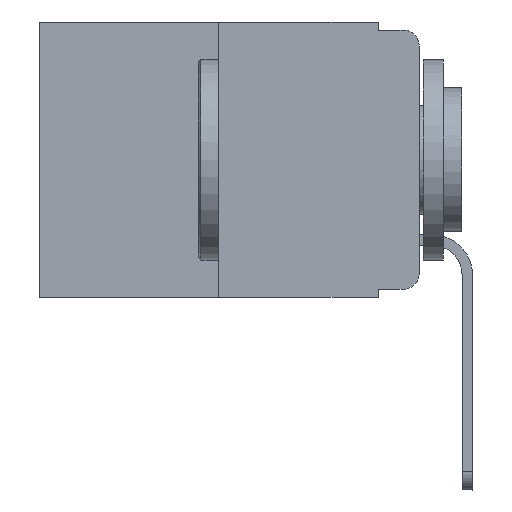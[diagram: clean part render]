
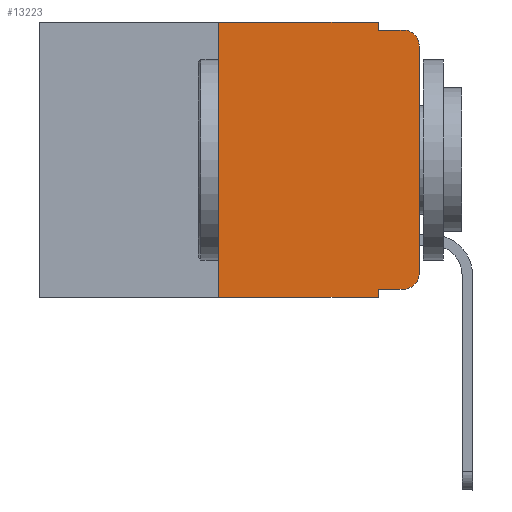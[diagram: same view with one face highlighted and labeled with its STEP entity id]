
A CAD part, left-side view. The second image highlights one B-rep face of the part: STEP entity #13223.
In plain terms, the highlighted planar face has unit normal (-1, 0, 0).
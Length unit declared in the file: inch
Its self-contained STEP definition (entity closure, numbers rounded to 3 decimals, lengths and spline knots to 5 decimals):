
#84 = CARTESIAN_POINT ( 'NONE',  ( 0., 0.02, -0.313 ) ) ;
#465 = ORIENTED_EDGE ( 'NONE', *, *, #11410, .T. ) ;
#489 = AXIS2_PLACEMENT_3D ( 'NONE', #3176, #11035, #1625 ) ;
#527 = EDGE_CURVE ( 'NONE', #16009, #16680, #5585, .T. ) ;
#617 = VERTEX_POINT ( 'NONE', #17067 ) ;
#781 = EDGE_CURVE ( 'NONE', #16009, #13276, #4056, .T. ) ;
#790 = EDGE_LOOP ( 'NONE', ( #15350, #3037, #8178, #7291, #4586, #2804, #465, #12180, #9884, #7773 ) ) ;
#1035 = CARTESIAN_POINT ( 'NONE',  ( 0., 0., -0.03 ) ) ;
#1084 = CARTESIAN_POINT ( 'NONE',  ( 0., 0.051, -0.333 ) ) ;
#1417 = DIRECTION ( 'NONE',  ( 0., 0., -1. ) ) ;
#1625 = DIRECTION ( 'NONE',  ( 0., 0., -1. ) ) ;
#1684 = CARTESIAN_POINT ( 'NONE',  ( 0., 0.051, -0.333 ) ) ;
#1905 = CIRCLE ( 'NONE', #489, 0.02 ) ;
#2572 = DIRECTION ( 'NONE',  ( 0., 0., 1. ) ) ;
#2657 = EDGE_CURVE ( 'NONE', #7784, #9000, #7597, .T. ) ;
#2804 = ORIENTED_EDGE ( 'NONE', *, *, #6366, .F. ) ;
#3037 = ORIENTED_EDGE ( 'NONE', *, *, #5635, .T. ) ;
#3176 = CARTESIAN_POINT ( 'NONE',  ( 0., 0.02, -0.03 ) ) ;
#3271 = LINE ( 'NONE', #16456, #14441 ) ;
#3291 = AXIS2_PLACEMENT_3D ( 'NONE', #14202, #5093, #7713 ) ;
#3328 = VERTEX_POINT ( 'NONE', #7029 ) ;
#3570 = CARTESIAN_POINT ( 'NONE',  ( 0., 0.051, -0.343 ) ) ;
#3596 = CIRCLE ( 'NONE', #12473, 0.02 ) ;
#4056 = LINE ( 'NONE', #5470, #16793 ) ;
#4154 = LINE ( 'NONE', #9353, #15046 ) ;
#4251 = DIRECTION ( 'NONE',  ( 0., -1., 0. ) ) ;
#4451 = CARTESIAN_POINT ( 'NONE',  ( 0., 0.473, 0. ) ) ;
#4586 = ORIENTED_EDGE ( 'NONE', *, *, #13481, .F. ) ;
#4615 = DIRECTION ( 'NONE',  ( 0., 0., 1. ) ) ;
#5093 = DIRECTION ( 'NONE',  ( 1., 0., 0. ) ) ;
#5470 = CARTESIAN_POINT ( 'NONE',  ( 0., 0.051, 0. ) ) ;
#5585 = LINE ( 'NONE', #1684, #8979 ) ;
#5635 = EDGE_CURVE ( 'NONE', #13794, #3328, #1905, .T. ) ;
#5742 = CARTESIAN_POINT ( 'NONE',  ( 0., 0.051, -0.01 ) ) ;
#5751 = CARTESIAN_POINT ( 'NONE',  ( 0., 0., -0.313 ) ) ;
#6366 = EDGE_CURVE ( 'NONE', #10535, #617, #4154, .T. ) ;
#6478 = FACE_OUTER_BOUND ( 'NONE', #790, .T. ) ;
#6491 = EDGE_CURVE ( 'NONE', #16680, #13921, #3596, .T. ) ;
#7029 = CARTESIAN_POINT ( 'NONE',  ( 0., 0.02, -0.01 ) ) ;
#7243 = VECTOR ( 'NONE', #14005, 39.37008 ) ;
#7291 = ORIENTED_EDGE ( 'NONE', *, *, #2657, .F. ) ;
#7329 = VECTOR ( 'NONE', #15746, 39.37008 ) ;
#7597 = LINE ( 'NONE', #12945, #7329 ) ;
#7713 = DIRECTION ( 'NONE',  ( 0., 0., -1. ) ) ;
#7773 = ORIENTED_EDGE ( 'NONE', *, *, #6491, .T. ) ;
#7784 = VERTEX_POINT ( 'NONE', #13475 ) ;
#7862 = DIRECTION ( 'NONE',  ( 0., 0., -1. ) ) ;
#8178 = ORIENTED_EDGE ( 'NONE', *, *, #16227, .F. ) ;
#8612 = EDGE_CURVE ( 'NONE', #13921, #13794, #3271, .T. ) ;
#8979 = VECTOR ( 'NONE', #4251, 39.37008 ) ;
#9000 = VERTEX_POINT ( 'NONE', #11008 ) ;
#9042 = PLANE ( 'NONE',  #3291 ) ;
#9353 = CARTESIAN_POINT ( 'NONE',  ( 0., 0.25, 0. ) ) ;
#9535 = DIRECTION ( 'NONE',  ( -1., 0., 0. ) ) ;
#9884 = ORIENTED_EDGE ( 'NONE', *, *, #527, .T. ) ;
#10197 = CARTESIAN_POINT ( 'NONE',  ( 0., 0.02, -0.333 ) ) ;
#10535 = VERTEX_POINT ( 'NONE', #11641 ) ;
#11008 = CARTESIAN_POINT ( 'NONE',  ( 0., 0.051, -0.01 ) ) ;
#11035 = DIRECTION ( 'NONE',  ( -1., 0., 0. ) ) ;
#11097 = DIRECTION ( 'NONE',  ( 0., -1., 0. ) ) ;
#11114 = LINE ( 'NONE', #4451, #7243 ) ;
#11410 = EDGE_CURVE ( 'NONE', #10535, #13276, #15534, .T. ) ;
#11641 = CARTESIAN_POINT ( 'NONE',  ( 0., 0.25, -0.343 ) ) ;
#12180 = ORIENTED_EDGE ( 'NONE', *, *, #781, .F. ) ;
#12250 = LINE ( 'NONE', #5742, #14181 ) ;
#12473 = AXIS2_PLACEMENT_3D ( 'NONE', #84, #9535, #1417 ) ;
#12945 = CARTESIAN_POINT ( 'NONE',  ( 0., 0.051, 0. ) ) ;
#13223 = ADVANCED_FACE ( 'NONE', ( #6478 ), #9042, .F. ) ;
#13276 = VERTEX_POINT ( 'NONE', #3570 ) ;
#13475 = CARTESIAN_POINT ( 'NONE',  ( 0., 0.051, 0. ) ) ;
#13481 = EDGE_CURVE ( 'NONE', #617, #7784, #11114, .T. ) ;
#13794 = VERTEX_POINT ( 'NONE', #1035 ) ;
#13921 = VERTEX_POINT ( 'NONE', #5751 ) ;
#14005 = DIRECTION ( 'NONE',  ( 0., -1., 0. ) ) ;
#14181 = VECTOR ( 'NONE', #11097, 39.37008 ) ;
#14202 = CARTESIAN_POINT ( 'NONE',  ( 0., 0.473, 0. ) ) ;
#14441 = VECTOR ( 'NONE', #4615, 39.37008 ) ;
#15046 = VECTOR ( 'NONE', #2572, 39.37008 ) ;
#15350 = ORIENTED_EDGE ( 'NONE', *, *, #8612, .T. ) ;
#15534 = LINE ( 'NONE', #16837, #17034 ) ;
#15627 = DIRECTION ( 'NONE',  ( 0., -1., 0. ) ) ;
#15746 = DIRECTION ( 'NONE',  ( 0., 0., -1. ) ) ;
#16009 = VERTEX_POINT ( 'NONE', #1084 ) ;
#16227 = EDGE_CURVE ( 'NONE', #9000, #3328, #12250, .T. ) ;
#16456 = CARTESIAN_POINT ( 'NONE',  ( 0., 0., 0. ) ) ;
#16680 = VERTEX_POINT ( 'NONE', #10197 ) ;
#16793 = VECTOR ( 'NONE', #7862, 39.37008 ) ;
#16837 = CARTESIAN_POINT ( 'NONE',  ( 0., 0.473, -0.343 ) ) ;
#17034 = VECTOR ( 'NONE', #15627, 39.37008 ) ;
#17067 = CARTESIAN_POINT ( 'NONE',  ( 0., 0.25, 0. ) ) ;
